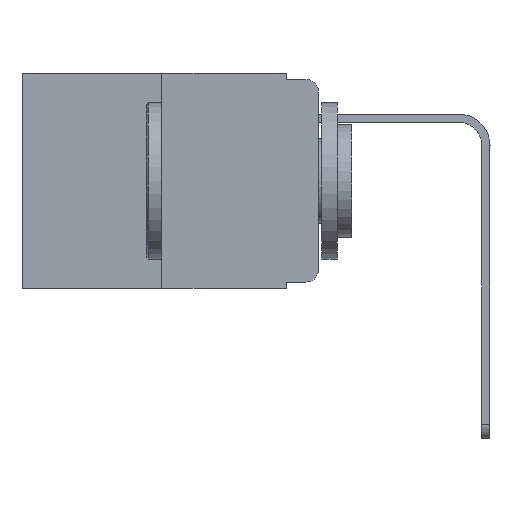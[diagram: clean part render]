
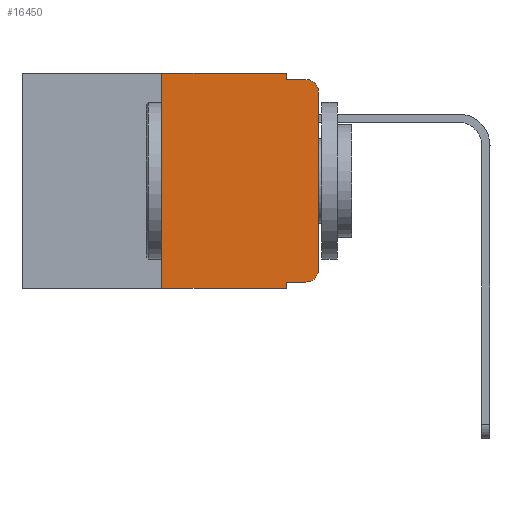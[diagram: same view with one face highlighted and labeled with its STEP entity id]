
A CAD part, left-side view. The second image highlights one B-rep face of the part: STEP entity #16450.
In plain terms, the highlighted planar face has unit normal (-1, 0, 0).
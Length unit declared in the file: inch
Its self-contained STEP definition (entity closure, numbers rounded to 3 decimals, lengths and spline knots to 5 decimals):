
#546 = VERTEX_POINT ( 'NONE', #10561 ) ;
#672 = LINE ( 'NONE', #9203, #17255 ) ;
#860 = AXIS2_PLACEMENT_3D ( 'NONE', #15142, #1219, #18063 ) ;
#1084 = LINE ( 'NONE', #5345, #10000 ) ;
#1219 = DIRECTION ( 'NONE',  ( -1., 0., 0. ) ) ;
#1607 = LINE ( 'NONE', #17842, #9882 ) ;
#1610 = ORIENTED_EDGE ( 'NONE', *, *, #4777, .F. ) ;
#1764 = CARTESIAN_POINT ( 'NONE',  ( 0., 0.02, -0.01 ) ) ;
#2214 = VECTOR ( 'NONE', #12919, 39.37008 ) ;
#2232 = VERTEX_POINT ( 'NONE', #9041 ) ;
#2267 = ORIENTED_EDGE ( 'NONE', *, *, #14359, .T. ) ;
#2409 = VERTEX_POINT ( 'NONE', #14079 ) ;
#2418 = DIRECTION ( 'NONE',  ( 0., -1., 0. ) ) ;
#3141 = CARTESIAN_POINT ( 'NONE',  ( 0., 0., 0. ) ) ;
#3337 = DIRECTION ( 'NONE',  ( 1., 0., 0. ) ) ;
#3545 = DIRECTION ( 'NONE',  ( 0., -1., 0. ) ) ;
#3921 = ORIENTED_EDGE ( 'NONE', *, *, #5053, .T. ) ;
#4185 = LINE ( 'NONE', #3141, #2214 ) ;
#4321 = ORIENTED_EDGE ( 'NONE', *, *, #17540, .T. ) ;
#4450 = CARTESIAN_POINT ( 'NONE',  ( 0., 0.02, -0.03 ) ) ;
#4777 = EDGE_CURVE ( 'NONE', #2409, #14991, #11837, .T. ) ;
#4820 = DIRECTION ( 'NONE',  ( 0., 0., -1. ) ) ;
#4877 = CARTESIAN_POINT ( 'NONE',  ( 0., 0.473, 0. ) ) ;
#5053 = EDGE_CURVE ( 'NONE', #11420, #5927, #4185, .T. ) ;
#5345 = CARTESIAN_POINT ( 'NONE',  ( 0., 0.051, -0.01 ) ) ;
#5350 = CARTESIAN_POINT ( 'NONE',  ( 0., 0., -0.03 ) ) ;
#5927 = VERTEX_POINT ( 'NONE', #5350 ) ;
#5957 = EDGE_CURVE ( 'NONE', #2409, #14343, #8048, .T. ) ;
#6001 = ORIENTED_EDGE ( 'NONE', *, *, #8860, .F. ) ;
#6534 = CARTESIAN_POINT ( 'NONE',  ( 0., 0., -0.313 ) ) ;
#6975 = LINE ( 'NONE', #13461, #8942 ) ;
#7080 = DIRECTION ( 'NONE',  ( 0., -1., 0. ) ) ;
#7600 = DIRECTION ( 'NONE',  ( -1., 0., 0. ) ) ;
#7643 = VERTEX_POINT ( 'NONE', #1764 ) ;
#8048 = LINE ( 'NONE', #10768, #10466 ) ;
#8286 = ORIENTED_EDGE ( 'NONE', *, *, #17756, .F. ) ;
#8361 = CARTESIAN_POINT ( 'NONE',  ( 0., 0.051, 0. ) ) ;
#8860 = EDGE_CURVE ( 'NONE', #14211, #7643, #1084, .T. ) ;
#8942 = VECTOR ( 'NONE', #9085, 39.37008 ) ;
#9041 = CARTESIAN_POINT ( 'NONE',  ( 0., 0.25, -0.343 ) ) ;
#9085 = DIRECTION ( 'NONE',  ( 0., 0., -1. ) ) ;
#9203 = CARTESIAN_POINT ( 'NONE',  ( 0., 0.25, 0. ) ) ;
#9882 = VECTOR ( 'NONE', #12346, 39.37008 ) ;
#10000 = VECTOR ( 'NONE', #7080, 39.37008 ) ;
#10081 = PLANE ( 'NONE',  #13578 ) ;
#10305 = EDGE_CURVE ( 'NONE', #14343, #11420, #15090, .T. ) ;
#10306 = ORIENTED_EDGE ( 'NONE', *, *, #12946, .F. ) ;
#10372 = AXIS2_PLACEMENT_3D ( 'NONE', #4450, #7600, #4820 ) ;
#10466 = VECTOR ( 'NONE', #2418, 39.37008 ) ;
#10561 = CARTESIAN_POINT ( 'NONE',  ( 0., 0.25, 0. ) ) ;
#10768 = CARTESIAN_POINT ( 'NONE',  ( 0., 0.051, -0.333 ) ) ;
#11017 = EDGE_LOOP ( 'NONE', ( #3921, #4321, #6001, #16743, #10306, #8286, #2267, #1610, #11714, #13071 ) ) ;
#11420 = VERTEX_POINT ( 'NONE', #6534 ) ;
#11631 = DIRECTION ( 'NONE',  ( 0., 0., -1. ) ) ;
#11714 = ORIENTED_EDGE ( 'NONE', *, *, #5957, .T. ) ;
#11837 = LINE ( 'NONE', #8361, #13599 ) ;
#11958 = DIRECTION ( 'NONE',  ( 0., 0., 1. ) ) ;
#12136 = LINE ( 'NONE', #4877, #17163 ) ;
#12346 = DIRECTION ( 'NONE',  ( 0., -1., 0. ) ) ;
#12919 = DIRECTION ( 'NONE',  ( 0., 0., 1. ) ) ;
#12946 = EDGE_CURVE ( 'NONE', #546, #13988, #12136, .T. ) ;
#13071 = ORIENTED_EDGE ( 'NONE', *, *, #10305, .T. ) ;
#13336 = CARTESIAN_POINT ( 'NONE',  ( 0., 0.051, -0.01 ) ) ;
#13461 = CARTESIAN_POINT ( 'NONE',  ( 0., 0.051, 0. ) ) ;
#13517 = CARTESIAN_POINT ( 'NONE',  ( 0., 0.02, -0.333 ) ) ;
#13578 = AXIS2_PLACEMENT_3D ( 'NONE', #15665, #3337, #11631 ) ;
#13599 = VECTOR ( 'NONE', #15596, 39.37008 ) ;
#13988 = VERTEX_POINT ( 'NONE', #15637 ) ;
#14079 = CARTESIAN_POINT ( 'NONE',  ( 0., 0.051, -0.333 ) ) ;
#14211 = VERTEX_POINT ( 'NONE', #13336 ) ;
#14343 = VERTEX_POINT ( 'NONE', #13517 ) ;
#14359 = EDGE_CURVE ( 'NONE', #2232, #14991, #1607, .T. ) ;
#14991 = VERTEX_POINT ( 'NONE', #18054 ) ;
#15090 = CIRCLE ( 'NONE', #860, 0.02 ) ;
#15142 = CARTESIAN_POINT ( 'NONE',  ( 0., 0.02, -0.313 ) ) ;
#15571 = FACE_OUTER_BOUND ( 'NONE', #11017, .T. ) ;
#15596 = DIRECTION ( 'NONE',  ( 0., 0., -1. ) ) ;
#15637 = CARTESIAN_POINT ( 'NONE',  ( 0., 0.051, 0. ) ) ;
#15665 = CARTESIAN_POINT ( 'NONE',  ( 0., 0.473, 0. ) ) ;
#15755 = CIRCLE ( 'NONE', #10372, 0.02 ) ;
#16450 = ADVANCED_FACE ( 'NONE', ( #15571 ), #10081, .F. ) ;
#16743 = ORIENTED_EDGE ( 'NONE', *, *, #17270, .F. ) ;
#17163 = VECTOR ( 'NONE', #3545, 39.37008 ) ;
#17255 = VECTOR ( 'NONE', #11958, 39.37008 ) ;
#17270 = EDGE_CURVE ( 'NONE', #13988, #14211, #6975, .T. ) ;
#17540 = EDGE_CURVE ( 'NONE', #5927, #7643, #15755, .T. ) ;
#17756 = EDGE_CURVE ( 'NONE', #2232, #546, #672, .T. ) ;
#17842 = CARTESIAN_POINT ( 'NONE',  ( 0., 0.473, -0.343 ) ) ;
#18054 = CARTESIAN_POINT ( 'NONE',  ( 0., 0.051, -0.343 ) ) ;
#18063 = DIRECTION ( 'NONE',  ( 0., 0., -1. ) ) ;
